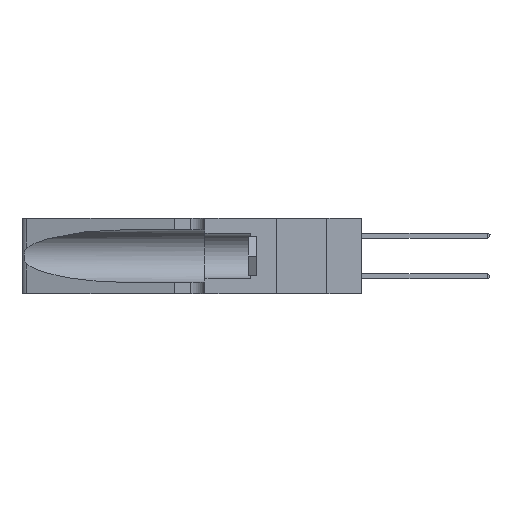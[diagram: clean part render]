
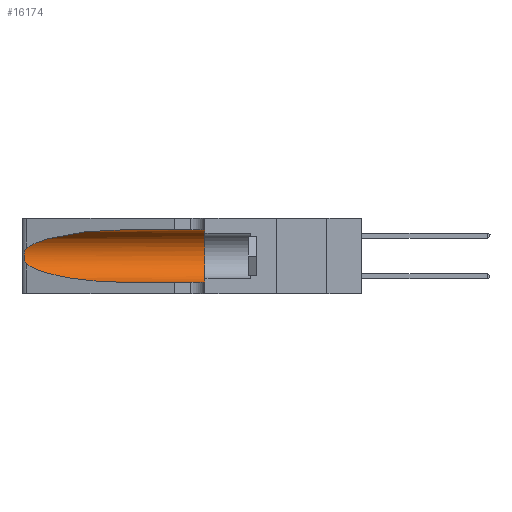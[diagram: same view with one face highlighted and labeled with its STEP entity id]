
A CAD part, left-side view. The second image highlights one B-rep face of the part: STEP entity #16174.
In plain terms, the highlighted cylindrical face has radius 3.308 mm (diameter 6.617 mm), a partial arc.
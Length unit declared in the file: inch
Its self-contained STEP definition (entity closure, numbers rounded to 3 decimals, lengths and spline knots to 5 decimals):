
#39 = CARTESIAN_POINT ( 'NONE',  ( 0.26018, 1.23835, 0.19895 ) ) ;
#114 = CARTESIAN_POINT ( 'NONE',  ( 0.26075, 1.23896, 0.178 ) ) ;
#200 = CARTESIAN_POINT ( 'NONE',  ( 0.25487, 1.22718, 0.22369 ) ) ;
#993 = FACE_OUTER_BOUND ( 'NONE', #8508, .T. ) ;
#1486 = DIRECTION ( 'NONE',  ( 0., -1., 0. ) ) ;
#1673 = CARTESIAN_POINT ( 'NONE',  ( 0.1305, 1.61858, 0.05475 ) ) ;
#2037 = DIRECTION ( 'NONE',  ( 0., 1., 0. ) ) ;
#2045 = VERTEX_POINT ( 'NONE', #17650 ) ;
#2126 = CARTESIAN_POINT ( 'NONE',  ( 0.2373, 1.15595, 0.28018 ) ) ;
#2308 = CARTESIAN_POINT ( 'NONE',  ( 0.26017, 1.23833, 0.17102 ) ) ;
#2339 = CARTESIAN_POINT ( 'NONE',  ( 0.25487, 1.22718, 0.22369 ) ) ;
#4157 = CARTESIAN_POINT ( 'NONE',  ( 0.1305, 0.72297, 0.31525 ) ) ;
#4349 = ORIENTED_EDGE ( 'NONE', *, *, #25335, .T. ) ;
#4571 =( BOUNDED_CURVE ( )  B_SPLINE_CURVE ( 3, ( #4157, #14544, #2126, #200 ),
 .UNSPECIFIED., .F., .F. ) 
 B_SPLINE_CURVE_WITH_KNOTS ( ( 4, 4 ),
 ( 1.5708, 2.84003 ),
 .UNSPECIFIED. ) 
 CURVE ( )  GEOMETRIC_REPRESENTATION_ITEM ( )  RATIONAL_B_SPLINE_CURVE ( ( 1., 0.87, 0.87, 1. ) ) 
 REPRESENTATION_ITEM ( '' )  );
#4781 = VECTOR ( 'NONE', #1486, 39.37008 ) ;
#5263 = LINE ( 'NONE', #1673, #13648 ) ;
#5624 = CARTESIAN_POINT ( 'NONE',  ( 0.1305, 0.35, 0.31525 ) ) ;
#6050 = LINE ( 'NONE', #22089, #4781 ) ;
#6211 = CARTESIAN_POINT ( 'NONE',  ( 0.25555, 1.22993, 0.14849 ) ) ;
#6467 = CARTESIAN_POINT ( 'NONE',  ( 0.25789, 1.23486, 0.15765 ) ) ;
#6562 = CARTESIAN_POINT ( 'NONE',  ( 0.2373, 1.15595, 0.08982 ) ) ;
#7040 = CARTESIAN_POINT ( 'NONE',  ( 0.1305, 0.72297, 0.05475 ) ) ;
#8222 = DIRECTION ( 'NONE',  ( 0., 0., 1. ) ) ;
#8508 = EDGE_LOOP ( 'NONE', ( #4349, #21674, #15549, #19967, #11201, #16332 ) ) ;
#8597 = CARTESIAN_POINT ( 'NONE',  ( 0.1305, 1.61858, 0.185 ) ) ;
#8663 = CARTESIAN_POINT ( 'NONE',  ( 0.25555, 1.22994, 0.2215 ) ) ;
#9276 = CARTESIAN_POINT ( 'NONE',  ( 0.18966, 0.96281, 0.05475 ) ) ;
#9878 = CARTESIAN_POINT ( 'NONE',  ( 0.1305, 0.35, 0.05475 ) ) ;
#10278 = CARTESIAN_POINT ( 'NONE',  ( 0.25639, 1.23184, 0.21858 ) ) ;
#10568 = EDGE_CURVE ( 'NONE', #16089, #26540, #6050, .T. ) ;
#10614 = CARTESIAN_POINT ( 'NONE',  ( 0.26075, 1.23896, 0.19203 ) ) ;
#11201 = ORIENTED_EDGE ( 'NONE', *, *, #25355, .F. ) ;
#11550 = VERTEX_POINT ( 'NONE', #9878 ) ;
#11549 = AXIS2_PLACEMENT_3D ( 'NONE', #24921, #2037, #8222 ) ;
#11831 = B_SPLINE_CURVE_WITH_KNOTS ( 'NONE', 3,
 ( #14728, #8663, #10278, #14545, #24840, #39, #10614, #114, #2308, #18576, #6467, #24751, #6211, #25103 ),
 .UNSPECIFIED., .F., .F.,
 ( 4, 2, 2, 2, 2, 2, 4 ),
 ( 0., 0.00027, 0.00053, 0.00107, 0.0016, 0.00187, 0.00214 ),
 .UNSPECIFIED. ) ;
#12292 = VERTEX_POINT ( 'NONE', #7040 ) ;
#13484 = EDGE_CURVE ( 'NONE', #12292, #11550, #5263, .T. ) ;
#13648 = VECTOR ( 'NONE', #26756, 39.37008 ) ;
#14544 = CARTESIAN_POINT ( 'NONE',  ( 0.18966, 0.96281, 0.31525 ) ) ;
#14545 = CARTESIAN_POINT ( 'NONE',  ( 0.25787, 1.23484, 0.2124 ) ) ;
#14728 = CARTESIAN_POINT ( 'NONE',  ( 0.25487, 1.22718, 0.22369 ) ) ;
#15549 = ORIENTED_EDGE ( 'NONE', *, *, #25649, .T. ) ;
#16089 = VERTEX_POINT ( 'NONE', #26705 ) ;
#16174 = ADVANCED_FACE ( 'NONE', ( #993 ), #18772, .F. ) ;
#16332 = ORIENTED_EDGE ( 'NONE', *, *, #10568, .F. ) ;
#17088 = AXIS2_PLACEMENT_3D ( 'NONE', #8597, #24777, #18603 ) ;
#17485 = CARTESIAN_POINT ( 'NONE',  ( 0.1305, 0.72297, 0.05475 ) ) ;
#17650 = CARTESIAN_POINT ( 'NONE',  ( 0.25487, 1.22718, 0.14631 ) ) ;
#18191 = VERTEX_POINT ( 'NONE', #2339 ) ;
#18576 = CARTESIAN_POINT ( 'NONE',  ( 0.25856, 1.23593, 0.16098 ) ) ;
#18603 = DIRECTION ( 'NONE',  ( 0., 0., -1. ) ) ;
#18715 = EDGE_CURVE ( 'NONE', #18191, #2045, #11831, .T. ) ;
#18772 = CYLINDRICAL_SURFACE ( 'NONE', #17088, 0.13025 ) ;
#19967 = ORIENTED_EDGE ( 'NONE', *, *, #13484, .T. ) ;
#21674 = ORIENTED_EDGE ( 'NONE', *, *, #18715, .T. ) ;
#22089 = CARTESIAN_POINT ( 'NONE',  ( 0.1305, 1.61858, 0.31525 ) ) ;
#23464 = CARTESIAN_POINT ( 'NONE',  ( 0.25487, 1.22718, 0.14631 ) ) ;
#24648 = CIRCLE ( 'NONE', #11549, 0.13025 ) ;
#24751 = CARTESIAN_POINT ( 'NONE',  ( 0.25639, 1.23186, 0.15144 ) ) ;
#24777 = DIRECTION ( 'NONE',  ( 0., -1., 0. ) ) ;
#24840 = CARTESIAN_POINT ( 'NONE',  ( 0.25854, 1.2359, 0.20912 ) ) ;
#24921 = CARTESIAN_POINT ( 'NONE',  ( 0.1305, 0.35, 0.185 ) ) ;
#25098 =( BOUNDED_CURVE ( )  B_SPLINE_CURVE ( 3, ( #23464, #6562, #9276, #17485 ),
 .UNSPECIFIED., .F., .F. ) 
 B_SPLINE_CURVE_WITH_KNOTS ( ( 4, 4 ),
 ( 3.44316, 4.71239 ),
 .UNSPECIFIED. ) 
 CURVE ( )  GEOMETRIC_REPRESENTATION_ITEM ( )  RATIONAL_B_SPLINE_CURVE ( ( 1., 0.87, 0.87, 1. ) ) 
 REPRESENTATION_ITEM ( '' )  );
#25103 = CARTESIAN_POINT ( 'NONE',  ( 0.25487, 1.22718, 0.14631 ) ) ;
#25335 = EDGE_CURVE ( 'NONE', #16089, #18191, #4571, .T. ) ;
#25355 = EDGE_CURVE ( 'NONE', #26540, #11550, #24648, .T. ) ;
#25649 = EDGE_CURVE ( 'NONE', #2045, #12292, #25098, .T. ) ;
#26540 = VERTEX_POINT ( 'NONE', #5624 ) ;
#26705 = CARTESIAN_POINT ( 'NONE',  ( 0.1305, 0.72297, 0.31525 ) ) ;
#26756 = DIRECTION ( 'NONE',  ( 0., -1., 0. ) ) ;
